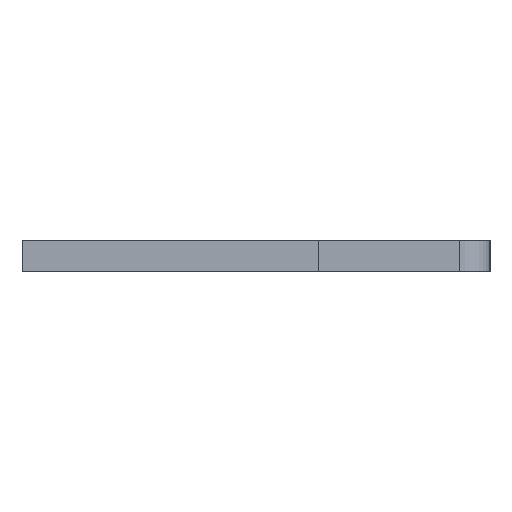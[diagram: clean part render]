
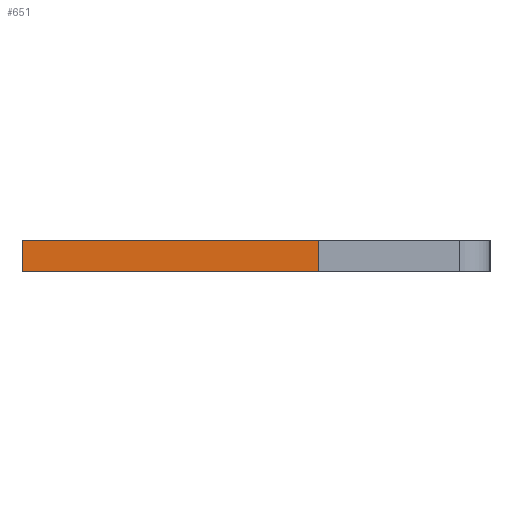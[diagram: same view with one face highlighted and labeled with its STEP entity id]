
A CAD part, left-side view. The second image highlights one B-rep face of the part: STEP entity #651.
In plain terms, the highlighted face is planar.
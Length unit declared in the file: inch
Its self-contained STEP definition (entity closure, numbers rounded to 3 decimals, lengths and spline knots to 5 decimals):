
#8 = PLANE ( 'NONE',  #234 ) ;
#57 = DIRECTION ( 'NONE',  ( 0., 1., 0. ) ) ;
#128 = LINE ( 'NONE', #1035, #200 ) ;
#139 = DIRECTION ( 'NONE',  ( 1., 0., 0. ) ) ;
#151 = EDGE_CURVE ( 'NONE', #312, #1266, #128, .T. ) ;
#163 = EDGE_CURVE ( 'NONE', #367, #312, #468, .T. ) ;
#168 = VECTOR ( 'NONE', #1462, 39.37008 ) ;
#200 = VECTOR ( 'NONE', #1329, 39.37008 ) ;
#234 = AXIS2_PLACEMENT_3D ( 'NONE', #1212, #1833, #139 ) ;
#243 = CARTESIAN_POINT ( 'NONE',  ( 0.01, -0.04, -0.04 ) ) ;
#312 = VERTEX_POINT ( 'NONE', #576 ) ;
#367 = VERTEX_POINT ( 'NONE', #1486 ) ;
#432 = CARTESIAN_POINT ( 'NONE',  ( 0.01, 0.15, -0.04 ) ) ;
#468 = LINE ( 'NONE', #432, #1766 ) ;
#471 = CARTESIAN_POINT ( 'NONE',  ( -0.01, -0.04, -0.04 ) ) ;
#576 = CARTESIAN_POINT ( 'NONE',  ( 0.01, 0.15, -0.04 ) ) ;
#584 = VERTEX_POINT ( 'NONE', #471 ) ;
#651 = ADVANCED_FACE ( 'NONE', ( #1158 ), #8, .F. ) ;
#805 = CARTESIAN_POINT ( 'NONE',  ( -0.01, 0.15, -0.04 ) ) ;
#814 = ORIENTED_EDGE ( 'NONE', *, *, #1597, .T. ) ;
#1032 = LINE ( 'NONE', #243, #168 ) ;
#1035 = CARTESIAN_POINT ( 'NONE',  ( 0.01, 0.15, -0.04 ) ) ;
#1081 = ORIENTED_EDGE ( 'NONE', *, *, #163, .F. ) ;
#1106 = EDGE_LOOP ( 'NONE', ( #814, #1528, #1081, #1336 ) ) ;
#1149 = CARTESIAN_POINT ( 'NONE',  ( -0.01, 0.15, -0.04 ) ) ;
#1158 = FACE_OUTER_BOUND ( 'NONE', #1106, .T. ) ;
#1212 = CARTESIAN_POINT ( 'NONE',  ( 0.01, 0.15, -0.04 ) ) ;
#1266 = VERTEX_POINT ( 'NONE', #805 ) ;
#1329 = DIRECTION ( 'NONE',  ( -1., 0., 0. ) ) ;
#1336 = ORIENTED_EDGE ( 'NONE', *, *, #1950, .T. ) ;
#1362 = VECTOR ( 'NONE', #57, 39.37008 ) ;
#1462 = DIRECTION ( 'NONE',  ( -1., 0., 0. ) ) ;
#1486 = CARTESIAN_POINT ( 'NONE',  ( 0.01, -0.04, -0.04 ) ) ;
#1528 = ORIENTED_EDGE ( 'NONE', *, *, #151, .F. ) ;
#1597 = EDGE_CURVE ( 'NONE', #584, #1266, #1762, .T. ) ;
#1762 = LINE ( 'NONE', #1149, #1362 ) ;
#1766 = VECTOR ( 'NONE', #1949, 39.37008 ) ;
#1833 = DIRECTION ( 'NONE',  ( 0., 0., 1. ) ) ;
#1949 = DIRECTION ( 'NONE',  ( 0., 1., 0. ) ) ;
#1950 = EDGE_CURVE ( 'NONE', #367, #584, #1032, .T. ) ;
